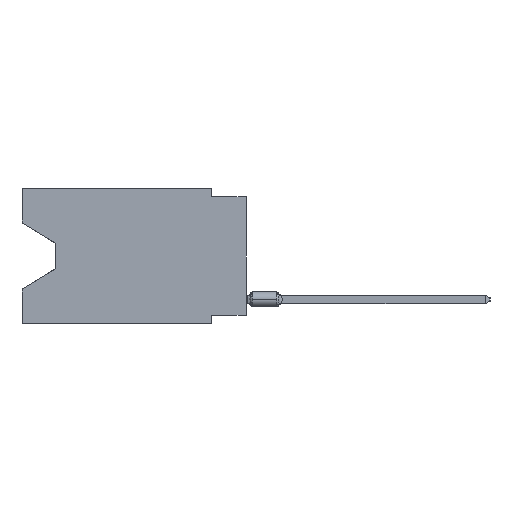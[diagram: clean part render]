
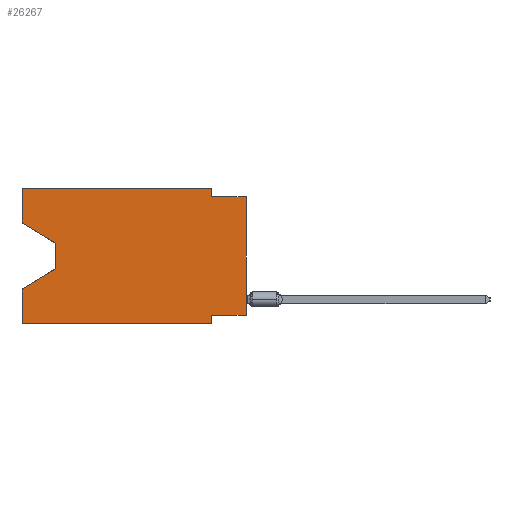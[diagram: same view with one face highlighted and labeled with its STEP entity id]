
A CAD part, left-side view. The second image highlights one B-rep face of the part: STEP entity #26267.
In plain terms, the highlighted planar face has unit normal (-1, 0, 0).
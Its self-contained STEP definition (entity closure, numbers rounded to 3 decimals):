
#1106 = LINE ( 'NONE', #60576, #70221 ) ;
#2139 = CARTESIAN_POINT ( 'NONE',  ( 0., 2.54, -9.906 ) ) ;
#3643 = CARTESIAN_POINT ( 'NONE',  ( 0., 16.383, 0. ) ) ;
#3660 = VERTEX_POINT ( 'NONE', #64233 ) ;
#4178 = CARTESIAN_POINT ( 'NONE',  ( 0., 16.383, -9.906 ) ) ;
#4849 = VERTEX_POINT ( 'NONE', #52027 ) ;
#5619 = DIRECTION ( 'NONE',  ( 0., 0.855, -0.519 ) ) ;
#5772 = VECTOR ( 'NONE', #20662, 1000. ) ;
#5880 = ORIENTED_EDGE ( 'NONE', *, *, #27595, .F. ) ;
#6112 = ORIENTED_EDGE ( 'NONE', *, *, #30765, .F. ) ;
#6980 = VECTOR ( 'NONE', #47430, 1000. ) ;
#7814 = DIRECTION ( 'NONE',  ( 0., 1., 0. ) ) ;
#8659 = EDGE_LOOP ( 'NONE', ( #65370, #60291, #9455, #24538, #48077, #26220, #5880, #64530, #70264, #26536, #44881, #6112 ) ) ;
#9455 = ORIENTED_EDGE ( 'NONE', *, *, #54337, .T. ) ;
#10984 = DIRECTION ( 'NONE',  ( 0., 0., -1. ) ) ;
#11576 = CARTESIAN_POINT ( 'NONE',  ( 0., 2.54, 0. ) ) ;
#11635 = DIRECTION ( 'NONE',  ( 0., 0., 1. ) ) ;
#11686 = VECTOR ( 'NONE', #13722, 1000. ) ;
#12053 = EDGE_CURVE ( 'NONE', #22673, #3660, #22563, .T. ) ;
#12866 = VERTEX_POINT ( 'NONE', #48873 ) ;
#13722 = DIRECTION ( 'NONE',  ( 0., -1., 0. ) ) ;
#14068 = CARTESIAN_POINT ( 'NONE',  ( 0., 16.383, 0. ) ) ;
#16728 = LINE ( 'NONE', #14068, #21398 ) ;
#18094 = CARTESIAN_POINT ( 'NONE',  ( 0., 0., -0.635 ) ) ;
#18430 = EDGE_CURVE ( 'NONE', #25071, #71132, #40556, .T. ) ;
#18908 = CARTESIAN_POINT ( 'NONE',  ( 0., 2.54, -9.906 ) ) ;
#20662 = DIRECTION ( 'NONE',  ( 0., 0., 1. ) ) ;
#21398 = VECTOR ( 'NONE', #48135, 1000. ) ;
#21723 = DIRECTION ( 'NONE',  ( 0., 0., -1. ) ) ;
#22083 = FACE_OUTER_BOUND ( 'NONE', #8659, .T. ) ;
#22563 = LINE ( 'NONE', #44305, #70014 ) ;
#22668 = VERTEX_POINT ( 'NONE', #11576 ) ;
#22673 = VERTEX_POINT ( 'NONE', #66318 ) ;
#22809 = DIRECTION ( 'NONE',  ( 0., -1., 0. ) ) ;
#24538 = ORIENTED_EDGE ( 'NONE', *, *, #57216, .F. ) ;
#24793 = CARTESIAN_POINT ( 'NONE',  ( 0., 0., -0.635 ) ) ;
#25071 = VERTEX_POINT ( 'NONE', #65593 ) ;
#25958 = CARTESIAN_POINT ( 'NONE',  ( 0., 16.383, -2.546 ) ) ;
#26220 = ORIENTED_EDGE ( 'NONE', *, *, #42823, .F. ) ;
#26267 = ADVANCED_FACE ( 'NONE', ( #22083 ), #44555, .F. ) ;
#26536 = ORIENTED_EDGE ( 'NONE', *, *, #40676, .F. ) ;
#27595 = EDGE_CURVE ( 'NONE', #43303, #47965, #62537, .T. ) ;
#30381 = LINE ( 'NONE', #52525, #6980 ) ;
#30661 = LINE ( 'NONE', #25958, #32423 ) ;
#30765 = EDGE_CURVE ( 'NONE', #4849, #35019, #16728, .T. ) ;
#32163 = VECTOR ( 'NONE', #57589, 1000. ) ;
#32423 = VECTOR ( 'NONE', #69482, 1000. ) ;
#34692 = CARTESIAN_POINT ( 'NONE',  ( 0., 2.54, 0. ) ) ;
#35019 = VERTEX_POINT ( 'NONE', #67007 ) ;
#37739 = VECTOR ( 'NONE', #56804, 1000. ) ;
#38043 = CARTESIAN_POINT ( 'NONE',  ( 0., 16.383, 0. ) ) ;
#40202 = LINE ( 'NONE', #55095, #43671 ) ;
#40556 = LINE ( 'NONE', #18094, #11686 ) ;
#40577 = LINE ( 'NONE', #2139, #32163 ) ;
#40676 = EDGE_CURVE ( 'NONE', #22668, #25071, #55740, .T. ) ;
#42823 = EDGE_CURVE ( 'NONE', #47965, #54092, #40577, .T. ) ;
#43303 = VERTEX_POINT ( 'NONE', #59674 ) ;
#43671 = VECTOR ( 'NONE', #22809, 1000. ) ;
#44305 = CARTESIAN_POINT ( 'NONE',  ( 0., 13.97, -4.013 ) ) ;
#44403 = LINE ( 'NONE', #49488, #62177 ) ;
#44555 = PLANE ( 'NONE',  #61550 ) ;
#44776 = EDGE_CURVE ( 'NONE', #4849, #22673, #30661, .T. ) ;
#44881 = ORIENTED_EDGE ( 'NONE', *, *, #48265, .F. ) ;
#47430 = DIRECTION ( 'NONE',  ( 0., -1., 0. ) ) ;
#47965 = VERTEX_POINT ( 'NONE', #48417 ) ;
#48077 = ORIENTED_EDGE ( 'NONE', *, *, #64723, .T. ) ;
#48135 = DIRECTION ( 'NONE',  ( 0., 0., 1. ) ) ;
#48265 = EDGE_CURVE ( 'NONE', #35019, #22668, #30381, .T. ) ;
#48417 = CARTESIAN_POINT ( 'NONE',  ( 0., 2.54, -9.271 ) ) ;
#48873 = CARTESIAN_POINT ( 'NONE',  ( 0., 16.383, -7.36 ) ) ;
#49488 = CARTESIAN_POINT ( 'NONE',  ( 0., 13.97, -5.893 ) ) ;
#52027 = CARTESIAN_POINT ( 'NONE',  ( 0., 16.383, -2.546 ) ) ;
#52525 = CARTESIAN_POINT ( 'NONE',  ( 0., 16.383, 0. ) ) ;
#54092 = VERTEX_POINT ( 'NONE', #18908 ) ;
#54337 = EDGE_CURVE ( 'NONE', #3660, #12866, #44403, .T. ) ;
#55095 = CARTESIAN_POINT ( 'NONE',  ( 0., 16.383, -9.906 ) ) ;
#55740 = LINE ( 'NONE', #34692, #37739 ) ;
#56804 = DIRECTION ( 'NONE',  ( 0., 0., -1. ) ) ;
#57100 = CARTESIAN_POINT ( 'NONE',  ( 0., 0., -9.271 ) ) ;
#57216 = EDGE_CURVE ( 'NONE', #57623, #12866, #70333, .T. ) ;
#57589 = DIRECTION ( 'NONE',  ( 0., 0., -1. ) ) ;
#57623 = VERTEX_POINT ( 'NONE', #4178 ) ;
#59674 = CARTESIAN_POINT ( 'NONE',  ( 0., 0., -9.271 ) ) ;
#60291 = ORIENTED_EDGE ( 'NONE', *, *, #12053, .T. ) ;
#60576 = CARTESIAN_POINT ( 'NONE',  ( 0., 0., 0. ) ) ;
#60987 = EDGE_CURVE ( 'NONE', #43303, #71132, #1106, .T. ) ;
#61550 = AXIS2_PLACEMENT_3D ( 'NONE', #38043, #66673, #21723 ) ;
#62177 = VECTOR ( 'NONE', #5619, 1000. ) ;
#62537 = LINE ( 'NONE', #57100, #70990 ) ;
#64233 = CARTESIAN_POINT ( 'NONE',  ( 0., 13.97, -5.893 ) ) ;
#64530 = ORIENTED_EDGE ( 'NONE', *, *, #60987, .T. ) ;
#64723 = EDGE_CURVE ( 'NONE', #57623, #54092, #40202, .T. ) ;
#65370 = ORIENTED_EDGE ( 'NONE', *, *, #44776, .T. ) ;
#65593 = CARTESIAN_POINT ( 'NONE',  ( 0., 2.54, -0.635 ) ) ;
#66318 = CARTESIAN_POINT ( 'NONE',  ( 0., 13.97, -4.013 ) ) ;
#66673 = DIRECTION ( 'NONE',  ( 1., 0., 0. ) ) ;
#67007 = CARTESIAN_POINT ( 'NONE',  ( 0., 16.383, 0. ) ) ;
#69482 = DIRECTION ( 'NONE',  ( 0., -0.855, -0.519 ) ) ;
#70014 = VECTOR ( 'NONE', #10984, 1000. ) ;
#70221 = VECTOR ( 'NONE', #11635, 1000. ) ;
#70264 = ORIENTED_EDGE ( 'NONE', *, *, #18430, .F. ) ;
#70333 = LINE ( 'NONE', #3643, #5772 ) ;
#70990 = VECTOR ( 'NONE', #7814, 1000. ) ;
#71132 = VERTEX_POINT ( 'NONE', #24793 ) ;
